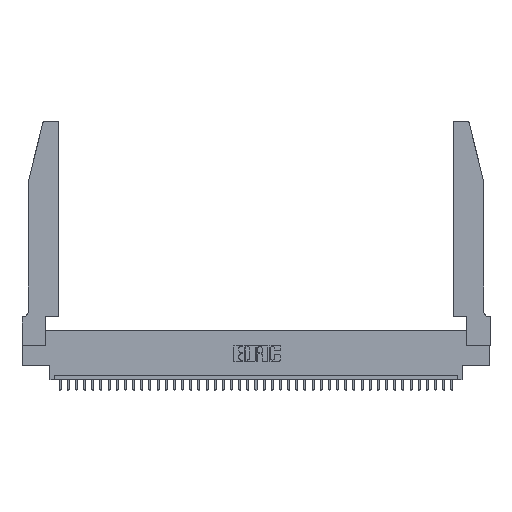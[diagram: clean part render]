
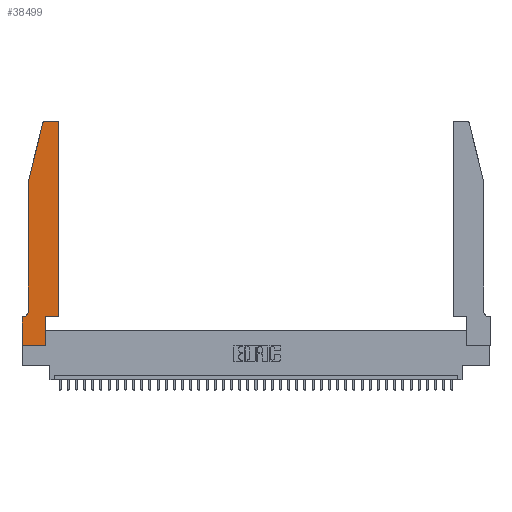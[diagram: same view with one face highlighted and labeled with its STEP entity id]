
A CAD part, top view. The second image highlights one B-rep face of the part: STEP entity #38499.
In plain terms, the highlighted planar face has unit normal (0, 0, 1).
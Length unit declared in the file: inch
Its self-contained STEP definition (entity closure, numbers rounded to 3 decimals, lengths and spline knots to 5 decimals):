
#104 = LINE ( 'NONE', #34232, #2104 ) ;
#1126 = CARTESIAN_POINT ( 'NONE',  ( 0.25487, 2.72718, 0.37 ) ) ;
#2104 = VECTOR ( 'NONE', #8812, 39.37008 ) ;
#3203 = LINE ( 'NONE', #20271, #35720 ) ;
#3250 = VERTEX_POINT ( 'NONE', #18657 ) ;
#3865 = CARTESIAN_POINT ( 'NONE',  ( 0.0755, 2., 0.37 ) ) ;
#4016 = EDGE_CURVE ( 'NONE', #13557, #40553, #5267, .T. ) ;
#5267 = LINE ( 'NONE', #12027, #28973 ) ;
#5888 = ORIENTED_EDGE ( 'NONE', *, *, #11212, .T. ) ;
#6025 = ORIENTED_EDGE ( 'NONE', *, *, #26908, .T. ) ;
#6918 = VERTEX_POINT ( 'NONE', #40663 ) ;
#7249 = CARTESIAN_POINT ( 'NONE',  ( 0., 0.35, 0.37 ) ) ;
#7267 = CARTESIAN_POINT ( 'NONE',  ( 0.2865, 0.35, 0.37 ) ) ;
#7337 = CARTESIAN_POINT ( 'NONE',  ( 0.284, 2.75, 0.37 ) ) ;
#7747 = DIRECTION ( 'NONE',  ( -1., 0., 0. ) ) ;
#7841 = DIRECTION ( 'NONE',  ( 0., 1., 0. ) ) ;
#8024 = CARTESIAN_POINT ( 'NONE',  ( 0.0755, 0.35, 0.37 ) ) ;
#8126 = VECTOR ( 'NONE', #20848, 39.37008 ) ;
#8158 = EDGE_CURVE ( 'NONE', #31246, #6918, #16304, .T. ) ;
#8618 = ORIENTED_EDGE ( 'NONE', *, *, #8158, .T. ) ;
#8812 = DIRECTION ( 'NONE',  ( 0., -1., 0. ) ) ;
#10314 = VERTEX_POINT ( 'NONE', #20109 ) ;
#10403 = DIRECTION ( 'NONE',  ( 1., 0., 0. ) ) ;
#10771 = DIRECTION ( 'NONE',  ( 1., 0., 0. ) ) ;
#11212 = EDGE_CURVE ( 'NONE', #40553, #10314, #27953, .T. ) ;
#11825 = EDGE_CURVE ( 'NONE', #18680, #13557, #13989, .T. ) ;
#11961 = CARTESIAN_POINT ( 'NONE',  ( 0.0755, 2., 0.37 ) ) ;
#12027 = CARTESIAN_POINT ( 'NONE',  ( 0.4505, 0.35, 0.37 ) ) ;
#12146 = ORIENTED_EDGE ( 'NONE', *, *, #26981, .T. ) ;
#12278 = ORIENTED_EDGE ( 'NONE', *, *, #15945, .T. ) ;
#13004 = VECTOR ( 'NONE', #14815, 39.37008 ) ;
#13194 = CARTESIAN_POINT ( 'NONE',  ( 0.284, 2.72, 0.37 ) ) ;
#13462 = DIRECTION ( 'NONE',  ( 1., 0., 0. ) ) ;
#13557 = VERTEX_POINT ( 'NONE', #7267 ) ;
#13989 = LINE ( 'NONE', #20298, #13004 ) ;
#14343 = CARTESIAN_POINT ( 'NONE',  ( 0., 0., 0.37 ) ) ;
#14815 = DIRECTION ( 'NONE',  ( 0., 1., 0. ) ) ;
#15126 = DIRECTION ( 'NONE',  ( -0.239, -0.971, 0. ) ) ;
#15672 = ORIENTED_EDGE ( 'NONE', *, *, #18746, .T. ) ;
#15945 = EDGE_CURVE ( 'NONE', #21585, #31246, #40795, .T. ) ;
#16304 = CIRCLE ( 'NONE', #20024, 0.07 ) ;
#16502 = ORIENTED_EDGE ( 'NONE', *, *, #11825, .T. ) ;
#16633 = DIRECTION ( 'NONE',  ( 0., 0., 1. ) ) ;
#16707 = ORIENTED_EDGE ( 'NONE', *, *, #29655, .T. ) ;
#17784 = AXIS2_PLACEMENT_3D ( 'NONE', #7249, #38605, #10403 ) ;
#17943 = CARTESIAN_POINT ( 'NONE',  ( 0., 0.35, 0.37 ) ) ;
#18281 = EDGE_CURVE ( 'NONE', #10314, #3250, #39359, .T. ) ;
#18657 = CARTESIAN_POINT ( 'NONE',  ( 0.4205, 2.75, 0.37 ) ) ;
#18680 = VERTEX_POINT ( 'NONE', #34395 ) ;
#18683 = ORIENTED_EDGE ( 'NONE', *, *, #4016, .T. ) ;
#18746 = EDGE_CURVE ( 'NONE', #23482, #22283, #25218, .T. ) ;
#20024 = AXIS2_PLACEMENT_3D ( 'NONE', #22251, #31957, #38012 ) ;
#20109 = CARTESIAN_POINT ( 'NONE',  ( 0.4505, 2.72, 0.37 ) ) ;
#20138 = FACE_OUTER_BOUND ( 'NONE', #38186, .T. ) ;
#20271 = CARTESIAN_POINT ( 'NONE',  ( 0.2605, 2.75, 0.37 ) ) ;
#20298 = CARTESIAN_POINT ( 'NONE',  ( 0.2865, 0.35, 0.37 ) ) ;
#20848 = DIRECTION ( 'NONE',  ( -1., 0., 0. ) ) ;
#21490 = AXIS2_PLACEMENT_3D ( 'NONE', #26560, #29685, #10771 ) ;
#21585 = VERTEX_POINT ( 'NONE', #11961 ) ;
#22089 = EDGE_CURVE ( 'NONE', #39778, #27256, #104, .T. ) ;
#22251 = CARTESIAN_POINT ( 'NONE',  ( 0.0055, 0.42, 0.37 ) ) ;
#22283 = VERTEX_POINT ( 'NONE', #1126 ) ;
#22542 = EDGE_CURVE ( 'NONE', #22283, #21585, #24895, .T. ) ;
#22778 = CARTESIAN_POINT ( 'NONE',  ( 0.0755, 0.42, 0.37 ) ) ;
#23482 = VERTEX_POINT ( 'NONE', #7337 ) ;
#23959 = LINE ( 'NONE', #8024, #8126 ) ;
#24895 = LINE ( 'NONE', #31219, #33132 ) ;
#25218 = CIRCLE ( 'NONE', #40740, 0.03 ) ;
#25469 = VECTOR ( 'NONE', #36352, 39.37008 ) ;
#26560 = CARTESIAN_POINT ( 'NONE',  ( 0.4205, 2.72, 0.37 ) ) ;
#26908 = EDGE_CURVE ( 'NONE', #27256, #18680, #33727, .T. ) ;
#26981 = EDGE_CURVE ( 'NONE', #6918, #39778, #23959, .T. ) ;
#27256 = VERTEX_POINT ( 'NONE', #39219 ) ;
#27953 = LINE ( 'NONE', #32712, #38644 ) ;
#28973 = VECTOR ( 'NONE', #31412, 39.37008 ) ;
#29655 = EDGE_CURVE ( 'NONE', #3250, #23482, #3203, .T. ) ;
#29685 = DIRECTION ( 'NONE',  ( 0., 0., 1. ) ) ;
#31219 = CARTESIAN_POINT ( 'NONE',  ( 0.0755, 2., 0.37 ) ) ;
#31246 = VERTEX_POINT ( 'NONE', #22778 ) ;
#31412 = DIRECTION ( 'NONE',  ( 1., 0., 0. ) ) ;
#31957 = DIRECTION ( 'NONE',  ( 0., 0., -1. ) ) ;
#32376 = VECTOR ( 'NONE', #38725, 39.37008 ) ;
#32712 = CARTESIAN_POINT ( 'NONE',  ( 0.4505, 0.35, 0.37 ) ) ;
#33132 = VECTOR ( 'NONE', #15126, 39.37008 ) ;
#33276 = ORIENTED_EDGE ( 'NONE', *, *, #22089, .T. ) ;
#33727 = LINE ( 'NONE', #14343, #25469 ) ;
#34232 = CARTESIAN_POINT ( 'NONE',  ( 0., 0., 0.37 ) ) ;
#34395 = CARTESIAN_POINT ( 'NONE',  ( 0.2865, 0., 0.37 ) ) ;
#35711 = PLANE ( 'NONE',  #17784 ) ;
#35720 = VECTOR ( 'NONE', #7747, 39.37008 ) ;
#36123 = ORIENTED_EDGE ( 'NONE', *, *, #18281, .T. ) ;
#36352 = DIRECTION ( 'NONE',  ( 1., 0., 0. ) ) ;
#36404 = ORIENTED_EDGE ( 'NONE', *, *, #22542, .T. ) ;
#37402 = CARTESIAN_POINT ( 'NONE',  ( 0.4505, 0.35, 0.37 ) ) ;
#38012 = DIRECTION ( 'NONE',  ( -1., 0., 0. ) ) ;
#38186 = EDGE_LOOP ( 'NONE', ( #16707, #15672, #36404, #12278, #8618, #12146, #33276, #6025, #16502, #18683, #5888, #36123 ) ) ;
#38499 = ADVANCED_FACE ( 'NONE', ( #20138 ), #35711, .T. ) ;
#38605 = DIRECTION ( 'NONE',  ( 0., 0., 1. ) ) ;
#38644 = VECTOR ( 'NONE', #7841, 39.37008 ) ;
#38725 = DIRECTION ( 'NONE',  ( 0., -1., 0. ) ) ;
#39219 = CARTESIAN_POINT ( 'NONE',  ( 0., 0., 0.37 ) ) ;
#39359 = CIRCLE ( 'NONE', #21490, 0.03 ) ;
#39778 = VERTEX_POINT ( 'NONE', #17943 ) ;
#40553 = VERTEX_POINT ( 'NONE', #37402 ) ;
#40663 = CARTESIAN_POINT ( 'NONE',  ( 0.0055, 0.35, 0.37 ) ) ;
#40740 = AXIS2_PLACEMENT_3D ( 'NONE', #13194, #16633, #13462 ) ;
#40795 = LINE ( 'NONE', #3865, #32376 ) ;
